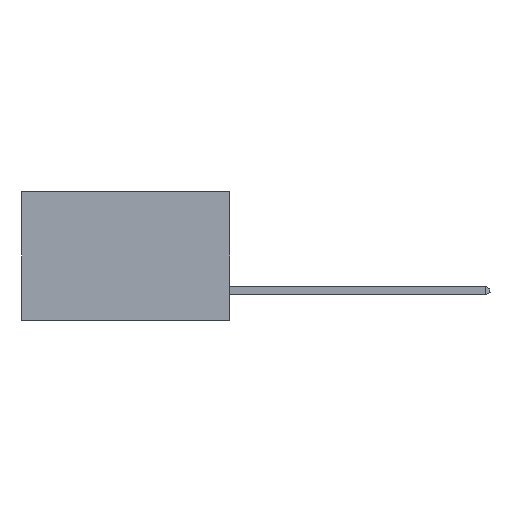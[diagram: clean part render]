
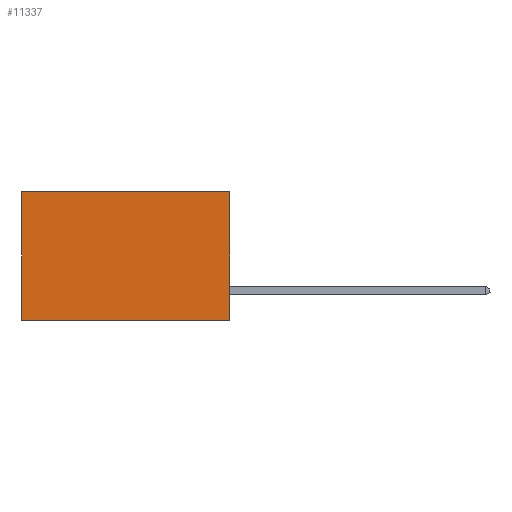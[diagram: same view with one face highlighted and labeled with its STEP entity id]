
A CAD part, left-side view. The second image highlights one B-rep face of the part: STEP entity #11337.
In plain terms, the highlighted planar face has unit normal (-1, 0, 0).
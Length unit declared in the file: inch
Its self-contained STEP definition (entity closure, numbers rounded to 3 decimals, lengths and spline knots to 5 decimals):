
#331 = CARTESIAN_POINT ( 'NONE',  ( 0.298, 0., 0. ) ) ;
#700 = DIRECTION ( 'NONE',  ( 0., 0., -1. ) ) ;
#860 = PLANE ( 'NONE',  #11129 ) ;
#878 = ORIENTED_EDGE ( 'NONE', *, *, #6597, .T. ) ;
#1309 = LINE ( 'NONE', #6968, #7555 ) ;
#1864 = CARTESIAN_POINT ( 'NONE',  ( 0.298, 0.6, -0.37 ) ) ;
#1975 = LINE ( 'NONE', #4226, #10860 ) ;
#2471 = FACE_OUTER_BOUND ( 'NONE', #12299, .T. ) ;
#3058 = ORIENTED_EDGE ( 'NONE', *, *, #12891, .F. ) ;
#3980 = VERTEX_POINT ( 'NONE', #331 ) ;
#4226 = CARTESIAN_POINT ( 'NONE',  ( 0.298, 0., 0. ) ) ;
#4288 = CARTESIAN_POINT ( 'NONE',  ( 0.298, 0., 0. ) ) ;
#5331 = VERTEX_POINT ( 'NONE', #14097 ) ;
#5675 = LINE ( 'NONE', #13418, #9422 ) ;
#6113 = EDGE_CURVE ( 'NONE', #10368, #8756, #5675, .T. ) ;
#6356 = CARTESIAN_POINT ( 'NONE',  ( 0.298, 0.6, 0. ) ) ;
#6597 = EDGE_CURVE ( 'NONE', #3980, #10368, #1309, .T. ) ;
#6968 = CARTESIAN_POINT ( 'NONE',  ( 0.298, 0., 0. ) ) ;
#7253 = DIRECTION ( 'NONE',  ( 0., 0., -1. ) ) ;
#7555 = VECTOR ( 'NONE', #9413, 39.37008 ) ;
#7991 = DIRECTION ( 'NONE',  ( 0., 0., -1. ) ) ;
#8192 = LINE ( 'NONE', #14938, #15362 ) ;
#8296 = ORIENTED_EDGE ( 'NONE', *, *, #6113, .T. ) ;
#8756 = VERTEX_POINT ( 'NONE', #1864 ) ;
#9413 = DIRECTION ( 'NONE',  ( 0., 1., 0. ) ) ;
#9422 = VECTOR ( 'NONE', #7253, 39.37008 ) ;
#10337 = ORIENTED_EDGE ( 'NONE', *, *, #11764, .F. ) ;
#10368 = VERTEX_POINT ( 'NONE', #6356 ) ;
#10860 = VECTOR ( 'NONE', #700, 39.37008 ) ;
#11129 = AXIS2_PLACEMENT_3D ( 'NONE', #4288, #13960, #7991 ) ;
#11337 = ADVANCED_FACE ( 'NONE', ( #2471 ), #860, .F. ) ;
#11764 = EDGE_CURVE ( 'NONE', #3980, #5331, #1975, .T. ) ;
#12299 = EDGE_LOOP ( 'NONE', ( #8296, #3058, #10337, #878 ) ) ;
#12891 = EDGE_CURVE ( 'NONE', #5331, #8756, #8192, .T. ) ;
#13418 = CARTESIAN_POINT ( 'NONE',  ( 0.298, 0.6, 0. ) ) ;
#13533 = DIRECTION ( 'NONE',  ( 0., 1., 0. ) ) ;
#13960 = DIRECTION ( 'NONE',  ( 1., 0., 0. ) ) ;
#14097 = CARTESIAN_POINT ( 'NONE',  ( 0.298, 0., -0.37 ) ) ;
#14938 = CARTESIAN_POINT ( 'NONE',  ( 0.298, 0., -0.37 ) ) ;
#15362 = VECTOR ( 'NONE', #13533, 39.37008 ) ;
